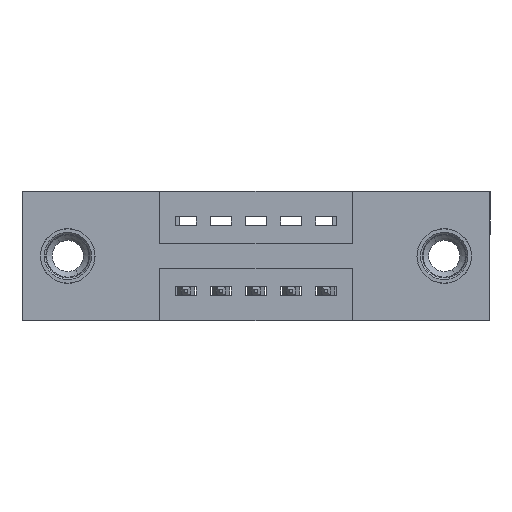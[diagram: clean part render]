
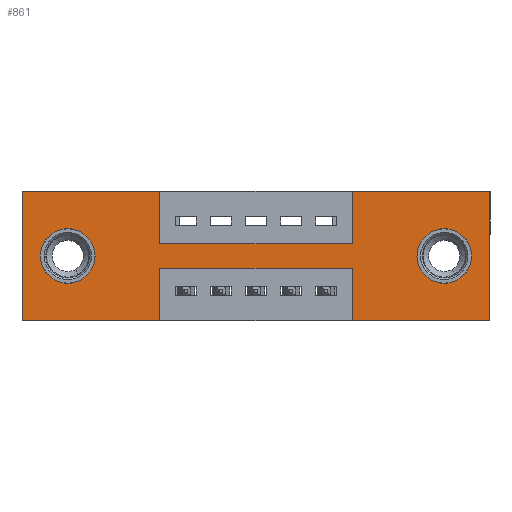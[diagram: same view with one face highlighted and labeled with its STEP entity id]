
A CAD part, front view. The second image highlights one B-rep face of the part: STEP entity #861.
In plain terms, the highlighted planar face has unit normal (0, -1, 0).
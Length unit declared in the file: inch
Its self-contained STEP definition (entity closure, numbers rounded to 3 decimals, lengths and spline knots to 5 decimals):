
#102 = ORIENTED_EDGE ( 'NONE', *, *, #5772, .T. ) ;
#233 = CARTESIAN_POINT ( 'NONE',  ( 0.3925, 0., 0. ) ) ;
#294 = LINE ( 'NONE', #1617, #2748 ) ;
#375 = VERTEX_POINT ( 'NONE', #5091 ) ;
#458 = EDGE_CURVE ( 'NONE', #1836, #7876, #2027, .T. ) ;
#567 = CARTESIAN_POINT ( 'NONE',  ( 0.13, 0., -0.107 ) ) ;
#646 = ORIENTED_EDGE ( 'NONE', *, *, #5425, .F. ) ;
#736 = LINE ( 'NONE', #6227, #13127 ) ;
#833 = EDGE_LOOP ( 'NONE', ( #5567, #3255 ) ) ;
#861 = ADVANCED_FACE ( 'NONE', ( #6589, #3668, #8561 ), #4256, .T. ) ;
#936 = CARTESIAN_POINT ( 'NONE',  ( 0.3925, 0., -0.37 ) ) ;
#982 = VERTEX_POINT ( 'NONE', #8069 ) ;
#1125 = DIRECTION ( 'NONE',  ( 0., 0., 1. ) ) ;
#1152 = CARTESIAN_POINT ( 'NONE',  ( 0., 0., 0. ) ) ;
#1183 = AXIS2_PLACEMENT_3D ( 'NONE', #7003, #5904, #7081 ) ;
#1261 = DIRECTION ( 'NONE',  ( 0., 0., -1. ) ) ;
#1617 = CARTESIAN_POINT ( 'NONE',  ( 0., 0., 0. ) ) ;
#1646 = ORIENTED_EDGE ( 'NONE', *, *, #13278, .F. ) ;
#1681 = DIRECTION ( 'NONE',  ( 0., 0., -1. ) ) ;
#1814 = CARTESIAN_POINT ( 'NONE',  ( 1.205, 0., -0.185 ) ) ;
#1836 = VERTEX_POINT ( 'NONE', #8853 ) ;
#1840 = EDGE_CURVE ( 'NONE', #5757, #6364, #4790, .T. ) ;
#1915 = CARTESIAN_POINT ( 'NONE',  ( 0.3925, 0., -0.15 ) ) ;
#1995 = AXIS2_PLACEMENT_3D ( 'NONE', #8456, #5293, #1125 ) ;
#2027 = LINE ( 'NONE', #8375, #11018 ) ;
#2046 = EDGE_CURVE ( 'NONE', #375, #6711, #8698, .T. ) ;
#2202 = DIRECTION ( 'NONE',  ( -1., 0., 0. ) ) ;
#2230 = VERTEX_POINT ( 'NONE', #4232 ) ;
#2373 = ORIENTED_EDGE ( 'NONE', *, *, #7907, .F. ) ;
#2407 = CARTESIAN_POINT ( 'NONE',  ( 0.9425, 0., -0.15 ) ) ;
#2434 = VERTEX_POINT ( 'NONE', #5994 ) ;
#2647 = EDGE_LOOP ( 'NONE', ( #102, #6033 ) ) ;
#2748 = VECTOR ( 'NONE', #7791, 39.37008 ) ;
#2765 = ORIENTED_EDGE ( 'NONE', *, *, #8176, .F. ) ;
#3178 = DIRECTION ( 'NONE',  ( 0., 0., 1. ) ) ;
#3255 = ORIENTED_EDGE ( 'NONE', *, *, #5314, .T. ) ;
#3668 = FACE_BOUND ( 'NONE', #2647, .T. ) ;
#3976 = VERTEX_POINT ( 'NONE', #9901 ) ;
#4020 = VECTOR ( 'NONE', #5890, 39.37008 ) ;
#4033 = VERTEX_POINT ( 'NONE', #6787 ) ;
#4139 = VECTOR ( 'NONE', #10990, 39.37008 ) ;
#4223 = CARTESIAN_POINT ( 'NONE',  ( 0., 0., -0.37 ) ) ;
#4232 = CARTESIAN_POINT ( 'NONE',  ( 1.335, 0., 0. ) ) ;
#4256 = PLANE ( 'NONE',  #11695 ) ;
#4306 = DIRECTION ( 'NONE',  ( 0., 0., -1. ) ) ;
#4530 = ORIENTED_EDGE ( 'NONE', *, *, #12717, .F. ) ;
#4790 = LINE ( 'NONE', #11848, #4139 ) ;
#4835 = LINE ( 'NONE', #9869, #4020 ) ;
#5091 = CARTESIAN_POINT ( 'NONE',  ( 1.205, 0., -0.107 ) ) ;
#5113 = CARTESIAN_POINT ( 'NONE',  ( 0.9425, 0., -0.22 ) ) ;
#5128 = DIRECTION ( 'NONE',  ( 1., 0., 0. ) ) ;
#5204 = EDGE_CURVE ( 'NONE', #13356, #5757, #13205, .T. ) ;
#5221 = ORIENTED_EDGE ( 'NONE', *, *, #7070, .F. ) ;
#5280 = ORIENTED_EDGE ( 'NONE', *, *, #10321, .F. ) ;
#5293 = DIRECTION ( 'NONE',  ( 0., 1., 0. ) ) ;
#5314 = EDGE_CURVE ( 'NONE', #6711, #375, #8635, .T. ) ;
#5401 = VERTEX_POINT ( 'NONE', #567 ) ;
#5425 = EDGE_CURVE ( 'NONE', #7876, #4033, #294, .T. ) ;
#5567 = ORIENTED_EDGE ( 'NONE', *, *, #2046, .T. ) ;
#5608 = LINE ( 'NONE', #1915, #12480 ) ;
#5689 = VECTOR ( 'NONE', #8496, 39.37008 ) ;
#5757 = VERTEX_POINT ( 'NONE', #5113 ) ;
#5772 = EDGE_CURVE ( 'NONE', #5401, #2434, #9585, .T. ) ;
#5823 = VECTOR ( 'NONE', #9006, 39.37008 ) ;
#5890 = DIRECTION ( 'NONE',  ( 0., 0., 1. ) ) ;
#5904 = DIRECTION ( 'NONE',  ( 0., 1., 0. ) ) ;
#5908 = ORIENTED_EDGE ( 'NONE', *, *, #1840, .F. ) ;
#5994 = CARTESIAN_POINT ( 'NONE',  ( 0.13, 0., -0.263 ) ) ;
#6033 = ORIENTED_EDGE ( 'NONE', *, *, #9773, .T. ) ;
#6189 = CARTESIAN_POINT ( 'NONE',  ( 0.3925, 0., -0.22 ) ) ;
#6227 = CARTESIAN_POINT ( 'NONE',  ( 0., 0., 0. ) ) ;
#6364 = VERTEX_POINT ( 'NONE', #6189 ) ;
#6455 = AXIS2_PLACEMENT_3D ( 'NONE', #1814, #7982, #1681 ) ;
#6558 = ORIENTED_EDGE ( 'NONE', *, *, #7922, .F. ) ;
#6589 = FACE_BOUND ( 'NONE', #833, .T. ) ;
#6711 = VERTEX_POINT ( 'NONE', #8268 ) ;
#6755 = LINE ( 'NONE', #233, #8215 ) ;
#6787 = CARTESIAN_POINT ( 'NONE',  ( 0.3925, 0., 0. ) ) ;
#6994 = CARTESIAN_POINT ( 'NONE',  ( 0.3925, 0., -0.15 ) ) ;
#7003 = CARTESIAN_POINT ( 'NONE',  ( 0.13, 0., -0.185 ) ) ;
#7070 = EDGE_CURVE ( 'NONE', #12039, #982, #4835, .T. ) ;
#7081 = DIRECTION ( 'NONE',  ( 0., 0., 1. ) ) ;
#7103 = CARTESIAN_POINT ( 'NONE',  ( 0., 0., -0.37 ) ) ;
#7240 = LINE ( 'NONE', #7103, #11481 ) ;
#7300 = DIRECTION ( 'NONE',  ( 0., 0., -1. ) ) ;
#7791 = DIRECTION ( 'NONE',  ( 1., 0., 0. ) ) ;
#7876 = VERTEX_POINT ( 'NONE', #1152 ) ;
#7907 = EDGE_CURVE ( 'NONE', #13132, #12039, #5608, .T. ) ;
#7922 = EDGE_CURVE ( 'NONE', #13059, #1836, #7240, .T. ) ;
#7982 = DIRECTION ( 'NONE',  ( 0., 1., 0. ) ) ;
#7990 = ORIENTED_EDGE ( 'NONE', *, *, #5204, .F. ) ;
#8069 = CARTESIAN_POINT ( 'NONE',  ( 0.9425, 0., 0. ) ) ;
#8176 = EDGE_CURVE ( 'NONE', #4033, #13132, #6755, .T. ) ;
#8215 = VECTOR ( 'NONE', #1261, 39.37008 ) ;
#8268 = CARTESIAN_POINT ( 'NONE',  ( 1.205, 0., -0.263 ) ) ;
#8343 = AXIS2_PLACEMENT_3D ( 'NONE', #9334, #12587, #13542 ) ;
#8375 = CARTESIAN_POINT ( 'NONE',  ( 0., 0., 0. ) ) ;
#8389 = DIRECTION ( 'NONE',  ( 0., -1., 0. ) ) ;
#8436 = DIRECTION ( 'NONE',  ( -1., 0., 0. ) ) ;
#8456 = CARTESIAN_POINT ( 'NONE',  ( 0.13, 0., -0.185 ) ) ;
#8496 = DIRECTION ( 'NONE',  ( 0., 0., 1. ) ) ;
#8561 = FACE_OUTER_BOUND ( 'NONE', #12303, .T. ) ;
#8635 = CIRCLE ( 'NONE', #8343, 0.078 ) ;
#8698 = CIRCLE ( 'NONE', #6455, 0.078 ) ;
#8853 = CARTESIAN_POINT ( 'NONE',  ( 0., 0., -0.37 ) ) ;
#8863 = EDGE_CURVE ( 'NONE', #3976, #13356, #10996, .T. ) ;
#8877 = LINE ( 'NONE', #12832, #10646 ) ;
#9006 = DIRECTION ( 'NONE',  ( 0., 0., -1. ) ) ;
#9022 = ORIENTED_EDGE ( 'NONE', *, *, #458, .F. ) ;
#9334 = CARTESIAN_POINT ( 'NONE',  ( 1.205, 0., -0.185 ) ) ;
#9436 = CIRCLE ( 'NONE', #1183, 0.078 ) ;
#9585 = CIRCLE ( 'NONE', #1995, 0.078 ) ;
#9656 = ORIENTED_EDGE ( 'NONE', *, *, #8863, .F. ) ;
#9677 = VECTOR ( 'NONE', #2202, 39.37008 ) ;
#9773 = EDGE_CURVE ( 'NONE', #2434, #5401, #9436, .T. ) ;
#9869 = CARTESIAN_POINT ( 'NONE',  ( 0.9425, 0., 0. ) ) ;
#9901 = CARTESIAN_POINT ( 'NONE',  ( 1.335, 0., -0.37 ) ) ;
#10321 = EDGE_CURVE ( 'NONE', #6364, #13059, #11216, .T. ) ;
#10646 = VECTOR ( 'NONE', #4306, 39.37008 ) ;
#10990 = DIRECTION ( 'NONE',  ( -1., 0., 0. ) ) ;
#10996 = LINE ( 'NONE', #4223, #9677 ) ;
#11018 = VECTOR ( 'NONE', #3178, 39.37008 ) ;
#11216 = LINE ( 'NONE', #13095, #5823 ) ;
#11481 = VECTOR ( 'NONE', #8436, 39.37008 ) ;
#11541 = CARTESIAN_POINT ( 'NONE',  ( 0., 0., -0.37 ) ) ;
#11685 = CARTESIAN_POINT ( 'NONE',  ( 0.9425, 0., -0.37 ) ) ;
#11695 = AXIS2_PLACEMENT_3D ( 'NONE', #11541, #8389, #7300 ) ;
#11848 = CARTESIAN_POINT ( 'NONE',  ( 0.3925, 0., -0.22 ) ) ;
#12039 = VERTEX_POINT ( 'NONE', #2407 ) ;
#12303 = EDGE_LOOP ( 'NONE', ( #5280, #5908, #7990, #9656, #1646, #4530, #5221, #2373, #2765, #646, #9022, #6558 ) ) ;
#12409 = DIRECTION ( 'NONE',  ( 1., 0., 0. ) ) ;
#12480 = VECTOR ( 'NONE', #12409, 39.37008 ) ;
#12587 = DIRECTION ( 'NONE',  ( 0., 1., 0. ) ) ;
#12717 = EDGE_CURVE ( 'NONE', #982, #2230, #736, .T. ) ;
#12740 = CARTESIAN_POINT ( 'NONE',  ( 0.9425, 0., -0.37 ) ) ;
#12832 = CARTESIAN_POINT ( 'NONE',  ( 1.335, 0., 0. ) ) ;
#13059 = VERTEX_POINT ( 'NONE', #936 ) ;
#13095 = CARTESIAN_POINT ( 'NONE',  ( 0.3925, 0., -0.37 ) ) ;
#13127 = VECTOR ( 'NONE', #5128, 39.37008 ) ;
#13132 = VERTEX_POINT ( 'NONE', #6994 ) ;
#13205 = LINE ( 'NONE', #12740, #5689 ) ;
#13278 = EDGE_CURVE ( 'NONE', #2230, #3976, #8877, .T. ) ;
#13356 = VERTEX_POINT ( 'NONE', #11685 ) ;
#13542 = DIRECTION ( 'NONE',  ( 0., 0., -1. ) ) ;
